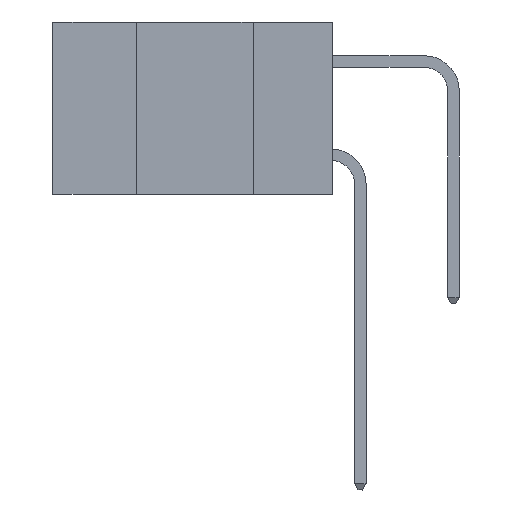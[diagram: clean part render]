
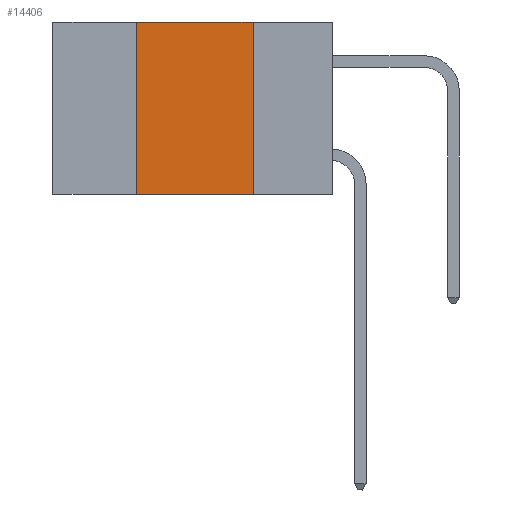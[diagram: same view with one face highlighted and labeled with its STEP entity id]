
A CAD part, left-side view. The second image highlights one B-rep face of the part: STEP entity #14406.
In plain terms, the highlighted planar face has unit normal (-1, 0, 0).
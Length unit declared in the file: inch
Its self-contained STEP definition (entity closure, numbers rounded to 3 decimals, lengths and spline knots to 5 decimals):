
#482 = CARTESIAN_POINT ( 'NONE',  ( 0., 0.42, 0. ) ) ;
#1509 = LINE ( 'NONE', #16025, #14657 ) ;
#3976 = ORIENTED_EDGE ( 'NONE', *, *, #20614, .F. ) ;
#4626 = PLANE ( 'NONE',  #13545 ) ;
#6478 = EDGE_CURVE ( 'NONE', #19889, #7760, #12647, .T. ) ;
#7245 = CARTESIAN_POINT ( 'NONE',  ( 0., 0.6, 0. ) ) ;
#7422 = DIRECTION ( 'NONE',  ( 0., 0., -1. ) ) ;
#7534 = CARTESIAN_POINT ( 'NONE',  ( 0., 0.17, 0. ) ) ;
#7644 = CARTESIAN_POINT ( 'NONE',  ( 0., 0.17, 0. ) ) ;
#7760 = VERTEX_POINT ( 'NONE', #482 ) ;
#9901 = DIRECTION ( 'NONE',  ( 0., 0., -1. ) ) ;
#11918 = VECTOR ( 'NONE', #7422, 39.37008 ) ;
#11956 = VERTEX_POINT ( 'NONE', #17235 ) ;
#12647 = LINE ( 'NONE', #31473, #18860 ) ;
#13545 = AXIS2_PLACEMENT_3D ( 'NONE', #7245, #25629, #9901 ) ;
#14406 = ADVANCED_FACE ( 'NONE', ( #21450 ), #4626, .F. ) ;
#14657 = VECTOR ( 'NONE', #18721, 39.37008 ) ;
#15083 = ORIENTED_EDGE ( 'NONE', *, *, #22073, .F. ) ;
#15777 = EDGE_CURVE ( 'NONE', #19889, #11956, #1509, .T. ) ;
#16025 = CARTESIAN_POINT ( 'NONE',  ( 0., 0.6, -0.37 ) ) ;
#17235 = CARTESIAN_POINT ( 'NONE',  ( 0., 0.17, -0.37 ) ) ;
#18434 = CARTESIAN_POINT ( 'NONE',  ( 0., 0.42, -0.37 ) ) ;
#18721 = DIRECTION ( 'NONE',  ( 0., -1., 0. ) ) ;
#18860 = VECTOR ( 'NONE', #22361, 39.37008 ) ;
#18949 = LINE ( 'NONE', #7534, #11918 ) ;
#19889 = VERTEX_POINT ( 'NONE', #18434 ) ;
#20614 = EDGE_CURVE ( 'NONE', #20666, #11956, #18949, .T. ) ;
#20666 = VERTEX_POINT ( 'NONE', #7644 ) ;
#21296 = ORIENTED_EDGE ( 'NONE', *, *, #6478, .F. ) ;
#21450 = FACE_OUTER_BOUND ( 'NONE', #22673, .T. ) ;
#22073 = EDGE_CURVE ( 'NONE', #7760, #20666, #28356, .T. ) ;
#22361 = DIRECTION ( 'NONE',  ( 0., 0., 1. ) ) ;
#22673 = EDGE_LOOP ( 'NONE', ( #3976, #15083, #21296, #23732 ) ) ;
#23134 = VECTOR ( 'NONE', #31237, 39.37008 ) ;
#23732 = ORIENTED_EDGE ( 'NONE', *, *, #15777, .T. ) ;
#25629 = DIRECTION ( 'NONE',  ( 1., 0., 0. ) ) ;
#26070 = CARTESIAN_POINT ( 'NONE',  ( 0., 0.6, 0. ) ) ;
#28356 = LINE ( 'NONE', #26070, #23134 ) ;
#31237 = DIRECTION ( 'NONE',  ( 0., -1., 0. ) ) ;
#31473 = CARTESIAN_POINT ( 'NONE',  ( 0., 0.42, 0. ) ) ;
